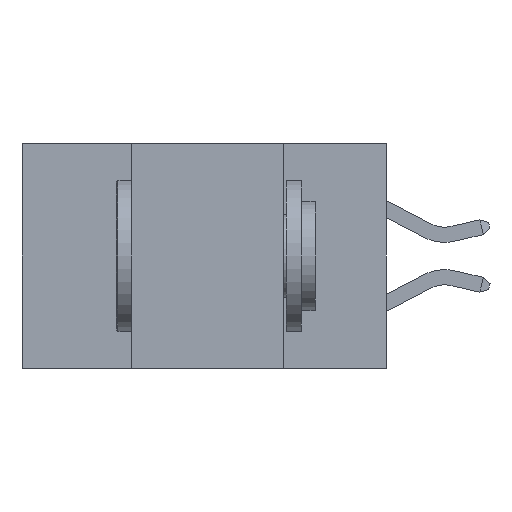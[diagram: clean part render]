
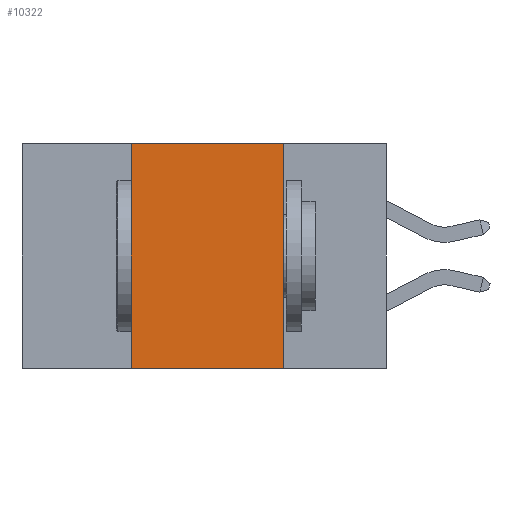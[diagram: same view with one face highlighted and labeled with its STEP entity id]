
A CAD part, left-side view. The second image highlights one B-rep face of the part: STEP entity #10322.
In plain terms, the highlighted planar face has unit normal (-1, 0, 0).
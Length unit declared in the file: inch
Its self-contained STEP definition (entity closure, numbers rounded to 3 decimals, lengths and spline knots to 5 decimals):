
#2429 = LINE ( 'NONE', #10427, #11403 ) ;
#3263 = VECTOR ( 'NONE', #17504, 39.37008 ) ;
#3327 = CARTESIAN_POINT ( 'NONE',  ( 0., 0.17, -0.37 ) ) ;
#4784 = EDGE_CURVE ( 'NONE', #18371, #8312, #13423, .T. ) ;
#4994 = FACE_OUTER_BOUND ( 'NONE', #15892, .T. ) ;
#5990 = EDGE_CURVE ( 'NONE', #18371, #11599, #2429, .T. ) ;
#7197 = EDGE_CURVE ( 'NONE', #8312, #21554, #21709, .T. ) ;
#7633 = DIRECTION ( 'NONE',  ( 1., 0., 0. ) ) ;
#8312 = VERTEX_POINT ( 'NONE', #16306 ) ;
#9914 = CARTESIAN_POINT ( 'NONE',  ( 0., 0.42, -0.37 ) ) ;
#10067 = CARTESIAN_POINT ( 'NONE',  ( 0., 0.6, 0. ) ) ;
#10322 = ADVANCED_FACE ( 'NONE', ( #4994 ), #12978, .F. ) ;
#10427 = CARTESIAN_POINT ( 'NONE',  ( 0., 0.6, -0.37 ) ) ;
#11403 = VECTOR ( 'NONE', #12231, 39.37008 ) ;
#11599 = VERTEX_POINT ( 'NONE', #18146 ) ;
#12013 = EDGE_CURVE ( 'NONE', #21554, #11599, #22064, .T. ) ;
#12231 = DIRECTION ( 'NONE',  ( 0., -1., 0. ) ) ;
#12467 = VECTOR ( 'NONE', #17097, 39.37008 ) ;
#12892 = VECTOR ( 'NONE', #16218, 39.37008 ) ;
#12978 = PLANE ( 'NONE',  #20244 ) ;
#13423 = LINE ( 'NONE', #21406, #12892 ) ;
#13609 = CARTESIAN_POINT ( 'NONE',  ( 0., 0.17, 0. ) ) ;
#15892 = EDGE_LOOP ( 'NONE', ( #21477, #21323, #21211, #20843 ) ) ;
#16218 = DIRECTION ( 'NONE',  ( 0., 0., 1. ) ) ;
#16306 = CARTESIAN_POINT ( 'NONE',  ( 0., 0.42, 0. ) ) ;
#17097 = DIRECTION ( 'NONE',  ( 0., -1., 0. ) ) ;
#17504 = DIRECTION ( 'NONE',  ( 0., 0., -1. ) ) ;
#18146 = CARTESIAN_POINT ( 'NONE',  ( 0., 0.17, -0.37 ) ) ;
#18183 = CARTESIAN_POINT ( 'NONE',  ( 0., 0.6, 0. ) ) ;
#18371 = VERTEX_POINT ( 'NONE', #9914 ) ;
#19928 = DIRECTION ( 'NONE',  ( 0., 0., -1. ) ) ;
#20244 = AXIS2_PLACEMENT_3D ( 'NONE', #18183, #7633, #19928 ) ;
#20843 = ORIENTED_EDGE ( 'NONE', *, *, #5990, .T. ) ;
#21211 = ORIENTED_EDGE ( 'NONE', *, *, #4784, .F. ) ;
#21323 = ORIENTED_EDGE ( 'NONE', *, *, #7197, .F. ) ;
#21406 = CARTESIAN_POINT ( 'NONE',  ( 0., 0.42, -0.37 ) ) ;
#21477 = ORIENTED_EDGE ( 'NONE', *, *, #12013, .F. ) ;
#21554 = VERTEX_POINT ( 'NONE', #13609 ) ;
#21709 = LINE ( 'NONE', #10067, #12467 ) ;
#22064 = LINE ( 'NONE', #3327, #3263 ) ;
